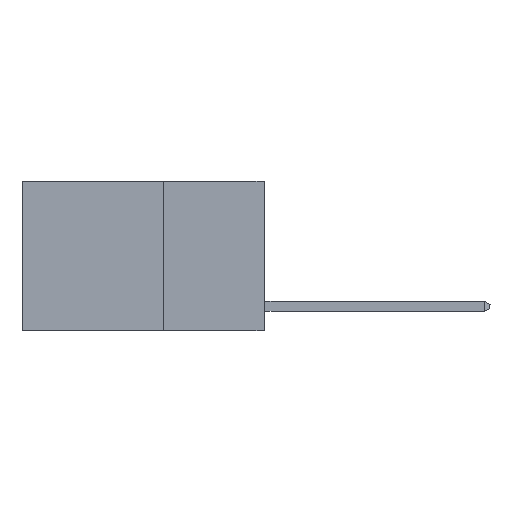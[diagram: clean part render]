
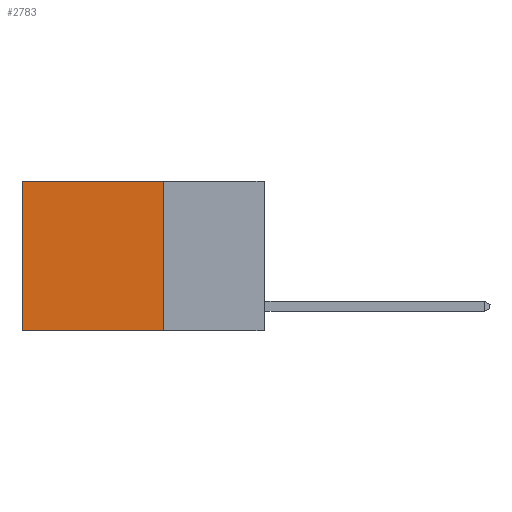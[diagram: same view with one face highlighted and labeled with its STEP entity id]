
A CAD part, left-side view. The second image highlights one B-rep face of the part: STEP entity #2783.
In plain terms, the highlighted planar face has unit normal (-1, 0, 0).
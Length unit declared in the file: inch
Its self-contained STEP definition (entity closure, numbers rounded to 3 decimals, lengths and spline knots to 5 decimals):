
#105 = CARTESIAN_POINT ( 'NONE',  ( 0.2625, 0.25, 0. ) ) ;
#773 = VECTOR ( 'NONE', #1601, 39.37008 ) ;
#1601 = DIRECTION ( 'NONE',  ( 0., 1., 0. ) ) ;
#1745 = ORIENTED_EDGE ( 'NONE', *, *, #15983, .T. ) ;
#2783 = ADVANCED_FACE ( 'NONE', ( #8362 ), #16397, .F. ) ;
#3509 = EDGE_CURVE ( 'NONE', #13391, #16517, #8112, .T. ) ;
#3611 = CARTESIAN_POINT ( 'NONE',  ( 0.2625, 0.6, 0. ) ) ;
#4100 = AXIS2_PLACEMENT_3D ( 'NONE', #6134, #19284, #7466 ) ;
#4665 = LINE ( 'NONE', #18971, #14178 ) ;
#4775 = VECTOR ( 'NONE', #4947, 39.37008 ) ;
#4947 = DIRECTION ( 'NONE',  ( 0., 1., 0. ) ) ;
#5363 = VECTOR ( 'NONE', #16489, 39.37008 ) ;
#5512 = DIRECTION ( 'NONE',  ( 0., 0., -1. ) ) ;
#5961 = CARTESIAN_POINT ( 'NONE',  ( 0.2625, 0.25, -0.37 ) ) ;
#6134 = CARTESIAN_POINT ( 'NONE',  ( 0.2625, 0.25, 0. ) ) ;
#6332 = ORIENTED_EDGE ( 'NONE', *, *, #8585, .F. ) ;
#7466 = DIRECTION ( 'NONE',  ( 0., 0., -1. ) ) ;
#8112 = LINE ( 'NONE', #105, #5363 ) ;
#8362 = FACE_OUTER_BOUND ( 'NONE', #9076, .T. ) ;
#8585 = EDGE_CURVE ( 'NONE', #16517, #10382, #9326, .T. ) ;
#9076 = EDGE_LOOP ( 'NONE', ( #13402, #6332, #9611, #1745 ) ) ;
#9326 = LINE ( 'NONE', #5961, #773 ) ;
#9501 = VERTEX_POINT ( 'NONE', #3611 ) ;
#9611 = ORIENTED_EDGE ( 'NONE', *, *, #3509, .F. ) ;
#10015 = CARTESIAN_POINT ( 'NONE',  ( 0.2625, 0.25, 0. ) ) ;
#10382 = VERTEX_POINT ( 'NONE', #13559 ) ;
#11722 = LINE ( 'NONE', #16936, #4775 ) ;
#13391 = VERTEX_POINT ( 'NONE', #10015 ) ;
#13402 = ORIENTED_EDGE ( 'NONE', *, *, #19080, .T. ) ;
#13559 = CARTESIAN_POINT ( 'NONE',  ( 0.2625, 0.6, -0.37 ) ) ;
#14178 = VECTOR ( 'NONE', #5512, 39.37008 ) ;
#15983 = EDGE_CURVE ( 'NONE', #13391, #9501, #11722, .T. ) ;
#16397 = PLANE ( 'NONE',  #4100 ) ;
#16489 = DIRECTION ( 'NONE',  ( 0., 0., -1. ) ) ;
#16517 = VERTEX_POINT ( 'NONE', #18368 ) ;
#16936 = CARTESIAN_POINT ( 'NONE',  ( 0.2625, 0.25, 0. ) ) ;
#18368 = CARTESIAN_POINT ( 'NONE',  ( 0.2625, 0.25, -0.37 ) ) ;
#18971 = CARTESIAN_POINT ( 'NONE',  ( 0.2625, 0.6, 0. ) ) ;
#19080 = EDGE_CURVE ( 'NONE', #9501, #10382, #4665, .T. ) ;
#19284 = DIRECTION ( 'NONE',  ( 1., 0., 0. ) ) ;
